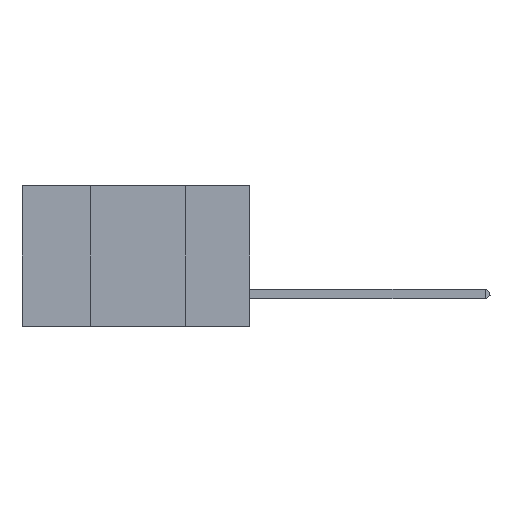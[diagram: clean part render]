
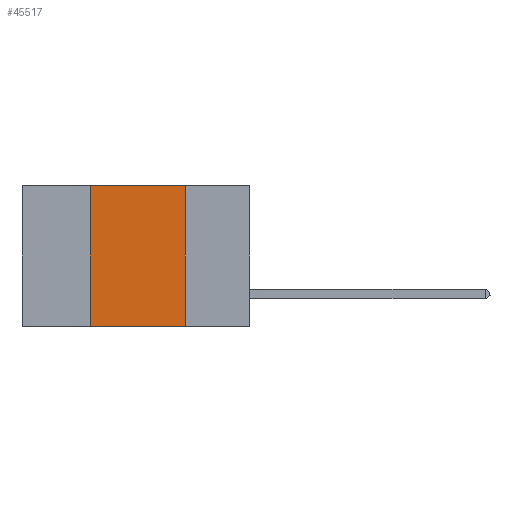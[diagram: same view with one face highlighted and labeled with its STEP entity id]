
A CAD part, left-side view. The second image highlights one B-rep face of the part: STEP entity #45517.
In plain terms, the highlighted planar face has unit normal (-1, 0, 0).
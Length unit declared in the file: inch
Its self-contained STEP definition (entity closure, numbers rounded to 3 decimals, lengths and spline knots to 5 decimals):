
#2602 = DIRECTION ( 'NONE',  ( 1., 0., 0. ) ) ;
#3766 = LINE ( 'NONE', #25264, #41776 ) ;
#6007 = VERTEX_POINT ( 'NONE', #18148 ) ;
#6408 = VERTEX_POINT ( 'NONE', #28876 ) ;
#6963 = DIRECTION ( 'NONE',  ( 0., -1., 0. ) ) ;
#9296 = AXIS2_PLACEMENT_3D ( 'NONE', #43048, #2602, #13703 ) ;
#12099 = CARTESIAN_POINT ( 'NONE',  ( 0., 0.6, -0.37 ) ) ;
#13703 = DIRECTION ( 'NONE',  ( 0., 0., -1. ) ) ;
#14266 = DIRECTION ( 'NONE',  ( 0., 0., 1. ) ) ;
#14482 = EDGE_LOOP ( 'NONE', ( #44145, #29323, #46928, #22133 ) ) ;
#14665 = EDGE_CURVE ( 'NONE', #6408, #6007, #26785, .T. ) ;
#16089 = EDGE_CURVE ( 'NONE', #39056, #6007, #18603, .T. ) ;
#18148 = CARTESIAN_POINT ( 'NONE',  ( 0., 0.17, -0.37 ) ) ;
#18603 = LINE ( 'NONE', #12099, #32448 ) ;
#19624 = DIRECTION ( 'NONE',  ( 0., 0., -1. ) ) ;
#22133 = ORIENTED_EDGE ( 'NONE', *, *, #16089, .T. ) ;
#22919 = DIRECTION ( 'NONE',  ( 0., -1., 0. ) ) ;
#25264 = CARTESIAN_POINT ( 'NONE',  ( 0., 0.42, 0. ) ) ;
#26785 = LINE ( 'NONE', #45738, #33712 ) ;
#28876 = CARTESIAN_POINT ( 'NONE',  ( 0., 0.17, 0. ) ) ;
#29323 = ORIENTED_EDGE ( 'NONE', *, *, #43902, .F. ) ;
#32187 = EDGE_CURVE ( 'NONE', #39056, #41175, #3766, .T. ) ;
#32448 = VECTOR ( 'NONE', #22919, 39.37008 ) ;
#33712 = VECTOR ( 'NONE', #19624, 39.37008 ) ;
#34483 = FACE_OUTER_BOUND ( 'NONE', #14482, .T. ) ;
#35188 = LINE ( 'NONE', #43884, #39259 ) ;
#35407 = CARTESIAN_POINT ( 'NONE',  ( 0., 0.42, 0. ) ) ;
#39056 = VERTEX_POINT ( 'NONE', #44481 ) ;
#39259 = VECTOR ( 'NONE', #6963, 39.37008 ) ;
#39667 = PLANE ( 'NONE',  #9296 ) ;
#41175 = VERTEX_POINT ( 'NONE', #35407 ) ;
#41776 = VECTOR ( 'NONE', #14266, 39.37008 ) ;
#43048 = CARTESIAN_POINT ( 'NONE',  ( 0., 0.6, 0. ) ) ;
#43884 = CARTESIAN_POINT ( 'NONE',  ( 0., 0.6, 0. ) ) ;
#43902 = EDGE_CURVE ( 'NONE', #41175, #6408, #35188, .T. ) ;
#44145 = ORIENTED_EDGE ( 'NONE', *, *, #14665, .F. ) ;
#44481 = CARTESIAN_POINT ( 'NONE',  ( 0., 0.42, -0.37 ) ) ;
#45517 = ADVANCED_FACE ( 'NONE', ( #34483 ), #39667, .F. ) ;
#45738 = CARTESIAN_POINT ( 'NONE',  ( 0., 0.17, 0. ) ) ;
#46928 = ORIENTED_EDGE ( 'NONE', *, *, #32187, .F. ) ;
